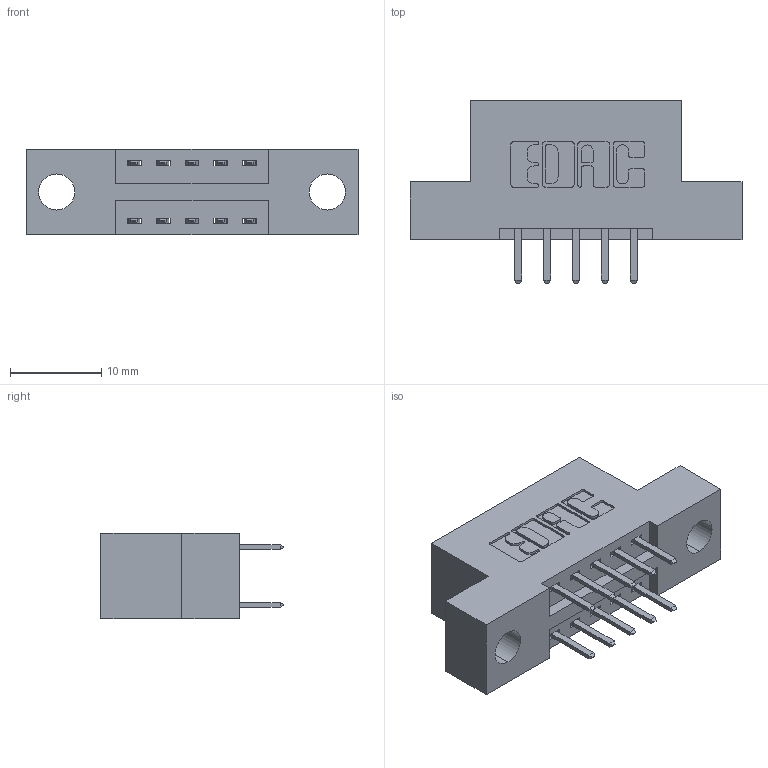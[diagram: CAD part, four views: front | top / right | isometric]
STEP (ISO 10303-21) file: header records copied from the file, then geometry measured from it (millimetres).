
FILE_DESCRIPTION (( 'STEP AP203' ), '1' );
FILE_NAME ('346-010-520-204.STEP', '2022-05-17T16:34:03', ( '' ), ( '' ), 'SwSTEP 2.0', 'SolidWorks 2020', '' );
FILE_SCHEMA (( 'CONFIG_CONTROL_DESIGN' ));
Length unit declared in the file: inch
Products named in the file (3): 345-292-001_345-293-120; 346-010-520-204; 346 Part_Flush Mounting Lugs - 0.156 Dia-TH
Assembly tree (11 placements, depth 2):
  346-010-520-204
    346 Part_Flush Mounting Lugs - 0.156 Dia-TH
    345-292-001_345-293-120  x10
Bounding box: 36.45 x 20.02 x 9.4 mm (x, y, z)
Volume: 3156.5 mm3; surface area: 3594.9 mm2
Topology: 11 solids, 11 shells, 696 faces, 1995 edges, 1302 vertices
Faces by surface type: plane 460, cylinder 236
Entity records: 8777 total; most frequent: CARTESIAN_POINT 1514, ORIENTED_EDGE 1434, DIRECTION 1373, EDGE_CURVE 717, VECTOR 561, LINE 561, VERTEX_POINT 474, AXIS2_PLACEMENT_3D 406
